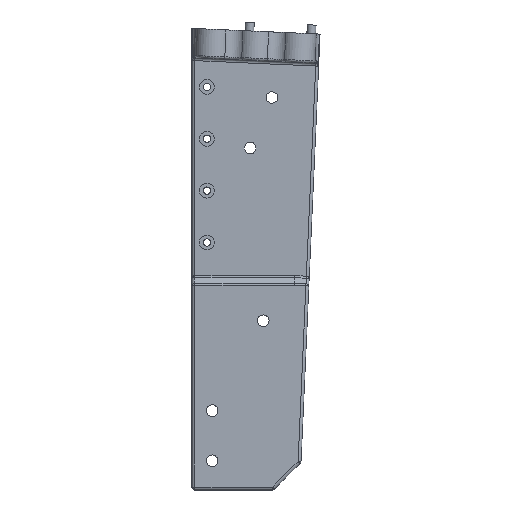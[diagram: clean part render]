
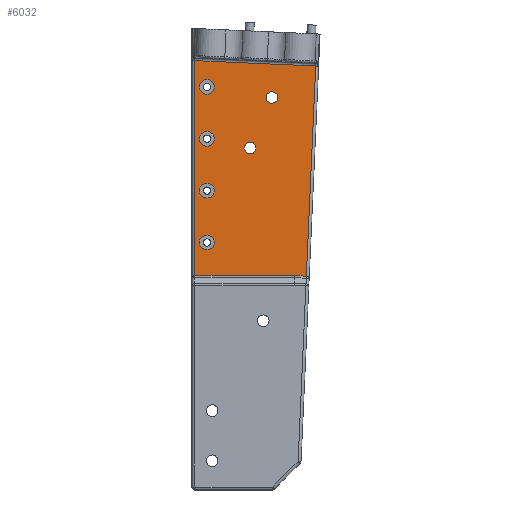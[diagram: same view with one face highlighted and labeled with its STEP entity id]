
A CAD part, left-side view. The second image highlights one B-rep face of the part: STEP entity #6032.
In plain terms, the highlighted planar face has unit normal (-1, 0, 0).
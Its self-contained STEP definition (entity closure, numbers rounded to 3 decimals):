
#40=ELLIPSE('',#6524,2.83,2.);
#218=FACE_BOUND('',#952,.T.);
#219=FACE_BOUND('',#953,.T.);
#220=FACE_BOUND('',#954,.T.);
#221=FACE_BOUND('',#955,.T.);
#222=FACE_BOUND('',#956,.T.);
#223=FACE_BOUND('',#957,.T.);
#290=PLANE('',#6580);
#566=FACE_OUTER_BOUND('',#951,.T.);
#951=EDGE_LOOP('',(#4712,#4713,#4714,#4715,#4716,#4717));
#952=EDGE_LOOP('',(#4718,#4719));
#953=EDGE_LOOP('',(#4720,#4721));
#954=EDGE_LOOP('',(#4722,#4723));
#955=EDGE_LOOP('',(#4724,#4725));
#956=EDGE_LOOP('',(#4726,#4727));
#957=EDGE_LOOP('',(#4728));
#1297=LINE('',#9393,#1826);
#1320=LINE('',#10007,#1849);
#1322=LINE('',#10034,#1851);
#1332=LINE('',#10078,#1861);
#1333=LINE('',#10080,#1862);
#1826=VECTOR('',#7329,10.);
#1849=VECTOR('',#7520,10.);
#1851=VECTOR('',#7532,10.);
#1861=VECTOR('',#7560,10.);
#1862=VECTOR('',#7563,10.);
#2255=CIRCLE('',#6259,2.54);
#2256=CIRCLE('',#6260,2.54);
#2260=CIRCLE('',#6266,2.54);
#2261=CIRCLE('',#6267,2.54);
#2265=CIRCLE('',#6273,2.54);
#2266=CIRCLE('',#6274,2.54);
#2270=CIRCLE('',#6280,2.54);
#2271=CIRCLE('',#6281,2.54);
#2447=CIRCLE('',#6581,2.);
#2448=CIRCLE('',#6582,2.);
#2449=CIRCLE('',#6583,2.);
#2529=VERTEX_POINT('',#8612);
#2530=VERTEX_POINT('',#8613);
#2534=VERTEX_POINT('',#8625);
#2535=VERTEX_POINT('',#8626);
#2539=VERTEX_POINT('',#8638);
#2540=VERTEX_POINT('',#8639);
#2544=VERTEX_POINT('',#8651);
#2545=VERTEX_POINT('',#8652);
#2700=VERTEX_POINT('',#9379);
#2704=VERTEX_POINT('',#9391);
#2785=VERTEX_POINT('',#9998);
#2788=VERTEX_POINT('',#10005);
#2790=VERTEX_POINT('',#10026);
#2792=VERTEX_POINT('',#10032);
#2818=VERTEX_POINT('',#10248);
#2819=VERTEX_POINT('',#10249);
#2820=VERTEX_POINT('',#10252);
#3097=EDGE_CURVE('',#2529,#2530,#2255,.T.);
#3098=EDGE_CURVE('',#2530,#2529,#2256,.T.);
#3103=EDGE_CURVE('',#2534,#2535,#2260,.T.);
#3104=EDGE_CURVE('',#2535,#2534,#2261,.T.);
#3109=EDGE_CURVE('',#2539,#2540,#2265,.T.);
#3110=EDGE_CURVE('',#2540,#2539,#2266,.T.);
#3115=EDGE_CURVE('',#2544,#2545,#2270,.T.);
#3116=EDGE_CURVE('',#2545,#2544,#2271,.T.);
#3334=EDGE_CURVE('',#2704,#2700,#1297,.T.);
#3447=EDGE_CURVE('',#2788,#2785,#1320,.T.);
#3450=EDGE_CURVE('',#2790,#2788,#40,.T.);
#3453=EDGE_CURVE('',#2792,#2790,#1322,.T.);
#3467=EDGE_CURVE('',#2785,#2704,#1332,.T.);
#3468=EDGE_CURVE('',#2700,#2792,#1333,.T.);
#3520=EDGE_CURVE('',#2818,#2819,#2447,.T.);
#3521=EDGE_CURVE('',#2819,#2818,#2448,.T.);
#3522=EDGE_CURVE('',#2820,#2820,#2449,.T.);
#4712=ORIENTED_EDGE('',*,*,#3334,.F.);
#4713=ORIENTED_EDGE('',*,*,#3467,.F.);
#4714=ORIENTED_EDGE('',*,*,#3447,.F.);
#4715=ORIENTED_EDGE('',*,*,#3450,.F.);
#4716=ORIENTED_EDGE('',*,*,#3453,.F.);
#4717=ORIENTED_EDGE('',*,*,#3468,.F.);
#4718=ORIENTED_EDGE('',*,*,#3097,.T.);
#4719=ORIENTED_EDGE('',*,*,#3098,.T.);
#4720=ORIENTED_EDGE('',*,*,#3103,.T.);
#4721=ORIENTED_EDGE('',*,*,#3104,.T.);
#4722=ORIENTED_EDGE('',*,*,#3109,.T.);
#4723=ORIENTED_EDGE('',*,*,#3110,.T.);
#4724=ORIENTED_EDGE('',*,*,#3115,.T.);
#4725=ORIENTED_EDGE('',*,*,#3116,.T.);
#4726=ORIENTED_EDGE('',*,*,#3520,.T.);
#4727=ORIENTED_EDGE('',*,*,#3521,.T.);
#4728=ORIENTED_EDGE('',*,*,#3522,.T.);
#6032=ADVANCED_FACE('',(#566,#218,#219,#220,#221,#222,#223),#290,.F.);
#6259=AXIS2_PLACEMENT_3D('',#8614,#6869,#6870);
#6260=AXIS2_PLACEMENT_3D('',#8615,#6871,#6872);
#6266=AXIS2_PLACEMENT_3D('',#8627,#6884,#6885);
#6267=AXIS2_PLACEMENT_3D('',#8628,#6886,#6887);
#6273=AXIS2_PLACEMENT_3D('',#8640,#6899,#6900);
#6274=AXIS2_PLACEMENT_3D('',#8641,#6901,#6902);
#6280=AXIS2_PLACEMENT_3D('',#8653,#6914,#6915);
#6281=AXIS2_PLACEMENT_3D('',#8654,#6916,#6917);
#6524=AXIS2_PLACEMENT_3D('',#10028,#7524,#7525);
#6580=AXIS2_PLACEMENT_3D('',#10247,#7687,#7688);
#6581=AXIS2_PLACEMENT_3D('',#10250,#7689,#7690);
#6582=AXIS2_PLACEMENT_3D('',#10251,#7691,#7692);
#6583=AXIS2_PLACEMENT_3D('',#10253,#7693,#7694);
#6869=DIRECTION('center_axis',(1.,0.,0.));
#6870=DIRECTION('ref_axis',(0.,0.,-1.));
#6871=DIRECTION('center_axis',(1.,0.,0.));
#6872=DIRECTION('ref_axis',(0.,0.,-1.));
#6884=DIRECTION('center_axis',(1.,0.,0.));
#6885=DIRECTION('ref_axis',(0.,0.,-1.));
#6886=DIRECTION('center_axis',(1.,0.,0.));
#6887=DIRECTION('ref_axis',(0.,0.,-1.));
#6899=DIRECTION('center_axis',(1.,0.,0.));
#6900=DIRECTION('ref_axis',(0.,0.,-1.));
#6901=DIRECTION('center_axis',(1.,0.,0.));
#6902=DIRECTION('ref_axis',(0.,0.,-1.));
#6914=DIRECTION('center_axis',(1.,0.,0.));
#6915=DIRECTION('ref_axis',(0.,0.,-1.));
#6916=DIRECTION('center_axis',(1.,0.,0.));
#6917=DIRECTION('ref_axis',(0.,0.,-1.));
#7329=DIRECTION('',(0.,-0.999,-0.044));
#7520=DIRECTION('',(0.,1.,0.));
#7524=DIRECTION('center_axis',(-1.,0.,0.));
#7525=DIRECTION('ref_axis',(0.,-0.044,0.999));
#7532=DIRECTION('',(0.,0.999,0.044));
#7560=DIRECTION('',(0.,0.,1.));
#7563=DIRECTION('',(0.,0.044,-0.999));
#7687=DIRECTION('center_axis',(1.,0.,0.));
#7688=DIRECTION('ref_axis',(0.,0.,-1.));
#7689=DIRECTION('center_axis',(1.,0.,0.));
#7690=DIRECTION('ref_axis',(0.,0.,1.));
#7691=DIRECTION('center_axis',(1.,0.,0.));
#7692=DIRECTION('ref_axis',(0.,0.,1.));
#7693=DIRECTION('center_axis',(1.,0.,0.));
#7694=DIRECTION('ref_axis',(0.,0.,1.));
#8612=CARTESIAN_POINT('',(-27.1,-5.186,100.046));
#8613=CARTESIAN_POINT('',(-27.1,-5.186,105.126));
#8614=CARTESIAN_POINT('Origin',(-27.1,-5.186,102.586));
#8615=CARTESIAN_POINT('Origin',(-27.1,-5.186,102.586));
#8625=CARTESIAN_POINT('',(-27.1,-5.186,117.826));
#8626=CARTESIAN_POINT('',(-27.1,-5.186,122.906));
#8627=CARTESIAN_POINT('Origin',(-27.1,-5.186,120.366));
#8628=CARTESIAN_POINT('Origin',(-27.1,-5.186,120.366));
#8638=CARTESIAN_POINT('',(-27.1,-5.186,82.266));
#8639=CARTESIAN_POINT('',(-27.1,-5.186,87.346));
#8640=CARTESIAN_POINT('Origin',(-27.1,-5.186,84.806));
#8641=CARTESIAN_POINT('Origin',(-27.1,-5.186,84.806));
#8651=CARTESIAN_POINT('',(-27.1,-5.186,135.606));
#8652=CARTESIAN_POINT('',(-27.1,-5.186,140.686));
#8653=CARTESIAN_POINT('Origin',(-27.1,-5.186,138.146));
#8654=CARTESIAN_POINT('Origin',(-27.1,-5.186,138.146));
#9379=CARTESIAN_POINT('',(-27.1,-42.475,145.293));
#9391=CARTESIAN_POINT('',(-27.1,-1.086,147.136));
#9393=CARTESIAN_POINT('',(-27.1,-22.548,146.181));
#9998=CARTESIAN_POINT('',(-27.1,-1.086,73.456));
#10005=CARTESIAN_POINT('',(-27.1,-35.224,73.456));
#10007=CARTESIAN_POINT('',(-27.1,-11.034,73.456));
#10026=CARTESIAN_POINT('',(-27.1,-35.287,73.454));
#10028=CARTESIAN_POINT('Origin',(-27.1,-35.161,70.627));
#10032=CARTESIAN_POINT('',(-27.1,-39.267,73.277));
#10034=CARTESIAN_POINT('',(-27.1,-27.812,73.787));
#10078=CARTESIAN_POINT('',(-27.1,-1.086,55.823));
#10080=CARTESIAN_POINT('',(-27.1,-39.739,83.86));
#10247=CARTESIAN_POINT('Origin',(-27.1,-22.024,111.646));
#10248=CARTESIAN_POINT('',(-27.1,-20.,115.2));
#10249=CARTESIAN_POINT('',(-27.1,-20.,119.2));
#10250=CARTESIAN_POINT('Origin',(-27.1,-20.,117.2));
#10251=CARTESIAN_POINT('Origin',(-27.1,-20.,117.2));
#10252=CARTESIAN_POINT('',(-27.1,-27.5,132.5));
#10253=CARTESIAN_POINT('Origin',(-27.1,-27.5,134.5));
